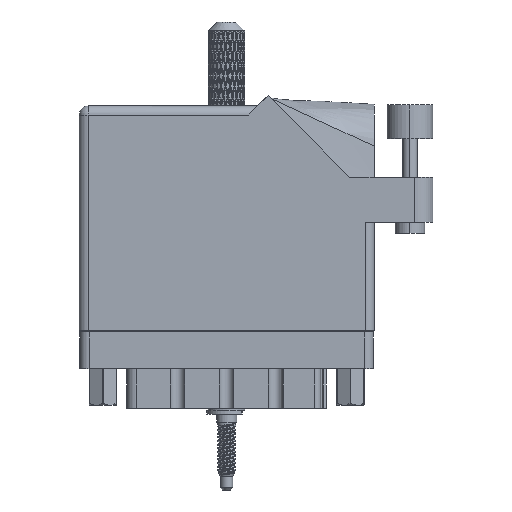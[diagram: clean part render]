
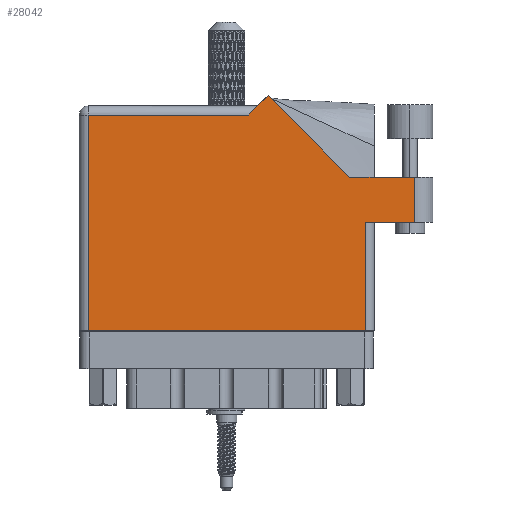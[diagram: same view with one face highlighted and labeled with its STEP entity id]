
A CAD part, front view. The second image highlights one B-rep face of the part: STEP entity #28042.
In plain terms, the highlighted face is planar.
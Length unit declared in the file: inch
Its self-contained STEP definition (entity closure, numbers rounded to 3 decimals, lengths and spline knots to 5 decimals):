
#2130 = EDGE_LOOP ( 'NONE', ( #41429, #21386, #66749, #44625, #56469, #48587, #16101, #34693, #10461 ) ) ;
#2705 = EDGE_CURVE ( 'NONE', #91248, #53624, #26488, .T. ) ;
#6252 = DIRECTION ( 'NONE',  ( -0.707, 0.707, 0. ) ) ;
#10461 = ORIENTED_EDGE ( 'NONE', *, *, #96710, .T. ) ;
#11809 = LINE ( 'NONE', #44021, #28592 ) ;
#16101 = ORIENTED_EDGE ( 'NONE', *, *, #28975, .T. ) ;
#21386 = ORIENTED_EDGE ( 'NONE', *, *, #24642, .T. ) ;
#24642 = EDGE_CURVE ( 'NONE', #46446, #71664, #33666, .T. ) ;
#24708 = CARTESIAN_POINT ( 'NONE',  ( 1.948, 0., 0. ) ) ;
#25233 = VECTOR ( 'NONE', #110196, 39.37008 ) ;
#26488 = LINE ( 'NONE', #72521, #32083 ) ;
#26901 = EDGE_CURVE ( 'NONE', #55380, #30317, #115492, .T. ) ;
#27037 = AXIS2_PLACEMENT_3D ( 'NONE', #99957, #28489, #81953 ) ;
#27375 = FACE_OUTER_BOUND ( 'NONE', #2130, .T. ) ;
#27656 = DIRECTION ( 'NONE',  ( -0.707, -0.707, 0. ) ) ;
#28042 = ADVANCED_FACE ( 'NONE', ( #27375 ), #37483, .F. ) ;
#28489 = DIRECTION ( 'NONE',  ( 0., 0., -1. ) ) ;
#28592 = VECTOR ( 'NONE', #53013, 39.37008 ) ;
#28975 = EDGE_CURVE ( 'NONE', #53624, #55380, #11809, .T. ) ;
#29512 = CARTESIAN_POINT ( 'NONE',  ( 0., 0., 0. ) ) ;
#30317 = VERTEX_POINT ( 'NONE', #24708 ) ;
#31056 = CARTESIAN_POINT ( 'NONE',  ( 1.28771, 1.60071, 0. ) ) ;
#32083 = VECTOR ( 'NONE', #37004, 39.37008 ) ;
#33666 = LINE ( 'NONE', #105710, #102096 ) ;
#34693 = ORIENTED_EDGE ( 'NONE', *, *, #26901, .T. ) ;
#37004 = DIRECTION ( 'NONE',  ( -1., 0., 0. ) ) ;
#37483 = PLANE ( 'NONE',  #27037 ) ;
#37720 = DIRECTION ( 'NONE',  ( 1., 0., 0. ) ) ;
#38909 = EDGE_CURVE ( 'NONE', #71113, #91248, #51664, .T. ) ;
#41429 = ORIENTED_EDGE ( 'NONE', *, *, #113450, .T. ) ;
#43616 = VERTEX_POINT ( 'NONE', #93332 ) ;
#43653 = EDGE_CURVE ( 'NONE', #43616, #71113, #63522, .T. ) ;
#43746 = VECTOR ( 'NONE', #95487, 39.37008 ) ;
#44021 = CARTESIAN_POINT ( 'NONE',  ( 0.062, 0., 0. ) ) ;
#44625 = ORIENTED_EDGE ( 'NONE', *, *, #43653, .T. ) ;
#45972 = CARTESIAN_POINT ( 'NONE',  ( 2.01, 0.737, 0. ) ) ;
#46096 = CARTESIAN_POINT ( 'NONE',  ( 1.948, 0.737, 0. ) ) ;
#46446 = VERTEX_POINT ( 'NONE', #108774 ) ;
#48587 = ORIENTED_EDGE ( 'NONE', *, *, #2705, .T. ) ;
#51664 = LINE ( 'NONE', #78805, #95010 ) ;
#52228 = DIRECTION ( 'NONE',  ( 0., 1., 0. ) ) ;
#53013 = DIRECTION ( 'NONE',  ( 0., -1., 0. ) ) ;
#53624 = VERTEX_POINT ( 'NONE', #108132 ) ;
#53748 = LINE ( 'NONE', #46096, #59338 ) ;
#55380 = VERTEX_POINT ( 'NONE', #59442 ) ;
#56469 = ORIENTED_EDGE ( 'NONE', *, *, #38909, .T. ) ;
#59338 = VECTOR ( 'NONE', #108554, 39.37008 ) ;
#59442 = CARTESIAN_POINT ( 'NONE',  ( 0.062, 0., 0. ) ) ;
#63522 = LINE ( 'NONE', #103833, #106918 ) ;
#66658 = VERTEX_POINT ( 'NONE', #94902 ) ;
#66749 = ORIENTED_EDGE ( 'NONE', *, *, #87667, .T. ) ;
#71113 = VERTEX_POINT ( 'NONE', #31056 ) ;
#71664 = VERTEX_POINT ( 'NONE', #97595 ) ;
#72521 = CARTESIAN_POINT ( 'NONE',  ( 0., 1.468, 0. ) ) ;
#78805 = CARTESIAN_POINT ( 'NONE',  ( 1.217, 1.53, 0. ) ) ;
#81953 = DIRECTION ( 'NONE',  ( -1., 0., 0. ) ) ;
#82473 = CARTESIAN_POINT ( 'NONE',  ( 2.41, 1.044, 0. ) ) ;
#85648 = LINE ( 'NONE', #45972, #43746 ) ;
#87667 = EDGE_CURVE ( 'NONE', #71664, #43616, #106207, .T. ) ;
#91248 = VERTEX_POINT ( 'NONE', #105823 ) ;
#93332 = CARTESIAN_POINT ( 'NONE',  ( 1.84442, 1.044, 0. ) ) ;
#94902 = CARTESIAN_POINT ( 'NONE',  ( 1.948, 0.737, 0. ) ) ;
#95010 = VECTOR ( 'NONE', #27656, 39.37008 ) ;
#95487 = DIRECTION ( 'NONE',  ( 1., 0., 0. ) ) ;
#96710 = EDGE_CURVE ( 'NONE', #30317, #66658, #53748, .T. ) ;
#97595 = CARTESIAN_POINT ( 'NONE',  ( 2.285, 1.044, 0. ) ) ;
#99957 = CARTESIAN_POINT ( 'NONE',  ( 0., 1.53, 0. ) ) ;
#101531 = VECTOR ( 'NONE', #37720, 39.37008 ) ;
#102096 = VECTOR ( 'NONE', #52228, 39.37008 ) ;
#103833 = CARTESIAN_POINT ( 'NONE',  ( 1.84442, 1.044, 0. ) ) ;
#105710 = CARTESIAN_POINT ( 'NONE',  ( 2.285, 1.044, 0. ) ) ;
#105823 = CARTESIAN_POINT ( 'NONE',  ( 1.155, 1.468, 0. ) ) ;
#106207 = LINE ( 'NONE', #82473, #25233 ) ;
#106918 = VECTOR ( 'NONE', #6252, 39.37008 ) ;
#108132 = CARTESIAN_POINT ( 'NONE',  ( 0.062, 1.468, 0. ) ) ;
#108554 = DIRECTION ( 'NONE',  ( 0., 1., 0. ) ) ;
#108774 = CARTESIAN_POINT ( 'NONE',  ( 2.285, 0.737, 0. ) ) ;
#110196 = DIRECTION ( 'NONE',  ( -1., 0., 0. ) ) ;
#113450 = EDGE_CURVE ( 'NONE', #66658, #46446, #85648, .T. ) ;
#115492 = LINE ( 'NONE', #29512, #101531 ) ;
